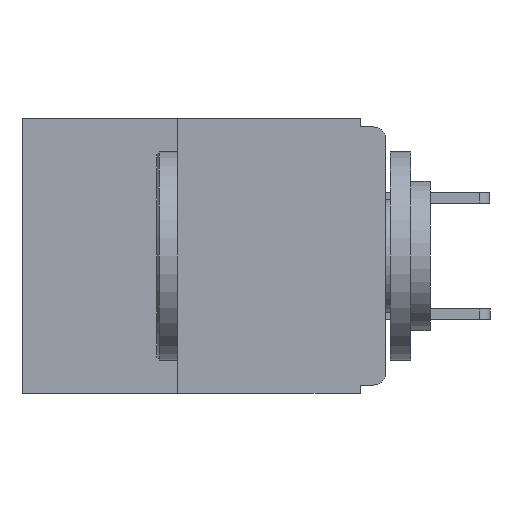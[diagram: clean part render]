
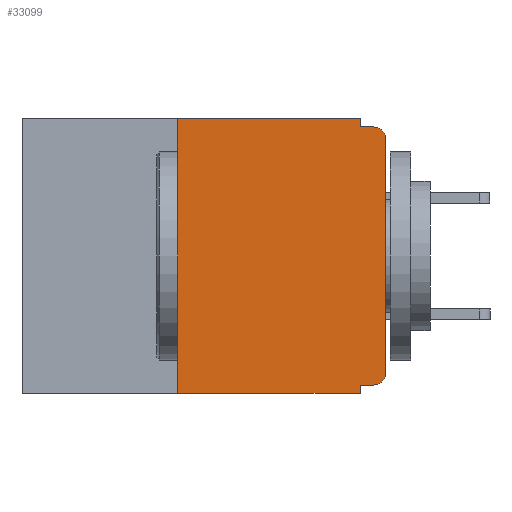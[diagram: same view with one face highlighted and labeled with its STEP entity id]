
A CAD part, left-side view. The second image highlights one B-rep face of the part: STEP entity #33099.
In plain terms, the highlighted planar face has unit normal (-1, 0, 0).
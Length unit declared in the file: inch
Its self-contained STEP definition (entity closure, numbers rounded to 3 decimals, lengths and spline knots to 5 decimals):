
#1001 = EDGE_CURVE ( 'NONE', #16274, #11754, #8063, .T. ) ;
#1783 = EDGE_CURVE ( 'NONE', #30344, #3031, #2550, .T. ) ;
#2550 = LINE ( 'NONE', #20270, #15804 ) ;
#3031 = VERTEX_POINT ( 'NONE', #18327 ) ;
#3470 = CARTESIAN_POINT ( 'NONE',  ( 0., 0.015, -0.01 ) ) ;
#3698 = AXIS2_PLACEMENT_3D ( 'NONE', #27168, #29694, #14377 ) ;
#3861 = CARTESIAN_POINT ( 'NONE',  ( 0., 0.437, 0. ) ) ;
#4147 = EDGE_CURVE ( 'NONE', #9978, #14993, #24090, .T. ) ;
#5062 = CARTESIAN_POINT ( 'NONE',  ( 0., 0.031, 0. ) ) ;
#5225 = DIRECTION ( 'NONE',  ( 0., 0., -1. ) ) ;
#5384 = AXIS2_PLACEMENT_3D ( 'NONE', #5745, #23966, #8425 ) ;
#5745 = CARTESIAN_POINT ( 'NONE',  ( 0., 0.015, -0.025 ) ) ;
#5998 = ORIENTED_EDGE ( 'NONE', *, *, #1001, .F. ) ;
#6214 = CARTESIAN_POINT ( 'NONE',  ( 0., 0., -0.025 ) ) ;
#6384 = VERTEX_POINT ( 'NONE', #3470 ) ;
#6578 = DIRECTION ( 'NONE',  ( 0., 0., 1. ) ) ;
#6771 = CARTESIAN_POINT ( 'NONE',  ( 0., 0.25, -0.33 ) ) ;
#7118 = EDGE_CURVE ( 'NONE', #16274, #3031, #19596, .T. ) ;
#7270 = VECTOR ( 'NONE', #7947, 39.37008 ) ;
#7947 = DIRECTION ( 'NONE',  ( 0., -1., 0. ) ) ;
#8063 = LINE ( 'NONE', #6771, #27885 ) ;
#8073 = CARTESIAN_POINT ( 'NONE',  ( 0., 0.437, -0.33 ) ) ;
#8425 = DIRECTION ( 'NONE',  ( 0., 0., -1. ) ) ;
#8981 = FACE_OUTER_BOUND ( 'NONE', #11424, .T. ) ;
#9074 = PLANE ( 'NONE',  #3698 ) ;
#9202 = CARTESIAN_POINT ( 'NONE',  ( 0., 0., -0.01 ) ) ;
#9669 = ORIENTED_EDGE ( 'NONE', *, *, #1783, .F. ) ;
#9970 = ORIENTED_EDGE ( 'NONE', *, *, #19701, .F. ) ;
#9978 = VERTEX_POINT ( 'NONE', #21602 ) ;
#10659 = CARTESIAN_POINT ( 'NONE',  ( 0., 0.031, -0.01 ) ) ;
#10823 = ORIENTED_EDGE ( 'NONE', *, *, #16907, .F. ) ;
#11361 = CARTESIAN_POINT ( 'NONE',  ( 0., 0.25, -0.33 ) ) ;
#11424 = EDGE_LOOP ( 'NONE', ( #22584, #19668, #19854, #10823, #9970, #5998, #25876, #9669, #19795, #16923 ) ) ;
#11754 = VERTEX_POINT ( 'NONE', #23821 ) ;
#11863 = DIRECTION ( 'NONE',  ( 0., -1., 0. ) ) ;
#12833 = DIRECTION ( 'NONE',  ( 0., 0., -1. ) ) ;
#12923 = EDGE_CURVE ( 'NONE', #19002, #6384, #29881, .T. ) ;
#13034 = DIRECTION ( 'NONE',  ( -1., 0., 0. ) ) ;
#13117 = CARTESIAN_POINT ( 'NONE',  ( 0., 0.015, -0.305 ) ) ;
#14040 = AXIS2_PLACEMENT_3D ( 'NONE', #13117, #13034, #12833 ) ;
#14279 = VECTOR ( 'NONE', #24736, 39.37008 ) ;
#14377 = DIRECTION ( 'NONE',  ( 0., 0., -1. ) ) ;
#14934 = LINE ( 'NONE', #19473, #26958 ) ;
#14993 = VERTEX_POINT ( 'NONE', #24313 ) ;
#15804 = VECTOR ( 'NONE', #5225, 39.37008 ) ;
#16274 = VERTEX_POINT ( 'NONE', #11361 ) ;
#16332 = EDGE_CURVE ( 'NONE', #9978, #30344, #14934, .T. ) ;
#16899 = LINE ( 'NONE', #21670, #22177 ) ;
#16907 = EDGE_CURVE ( 'NONE', #28744, #32203, #16899, .T. ) ;
#16923 = ORIENTED_EDGE ( 'NONE', *, *, #4147, .T. ) ;
#17728 = EDGE_CURVE ( 'NONE', #32203, #6384, #32751, .T. ) ;
#18327 = CARTESIAN_POINT ( 'NONE',  ( 0., 0.031, -0.33 ) ) ;
#19002 = VERTEX_POINT ( 'NONE', #6214 ) ;
#19473 = CARTESIAN_POINT ( 'NONE',  ( 0., 0., -0.32 ) ) ;
#19596 = LINE ( 'NONE', #8073, #7270 ) ;
#19668 = ORIENTED_EDGE ( 'NONE', *, *, #12923, .T. ) ;
#19701 = EDGE_CURVE ( 'NONE', #11754, #28744, #32994, .T. ) ;
#19795 = ORIENTED_EDGE ( 'NONE', *, *, #16332, .F. ) ;
#19854 = ORIENTED_EDGE ( 'NONE', *, *, #17728, .F. ) ;
#20270 = CARTESIAN_POINT ( 'NONE',  ( 0., 0.031, -0.33 ) ) ;
#20332 = DIRECTION ( 'NONE',  ( 0., 0., 1. ) ) ;
#21602 = CARTESIAN_POINT ( 'NONE',  ( 0., 0.015, -0.32 ) ) ;
#21670 = CARTESIAN_POINT ( 'NONE',  ( 0., 0.031, 0. ) ) ;
#22040 = DIRECTION ( 'NONE',  ( 0., 1., 0. ) ) ;
#22177 = VECTOR ( 'NONE', #24190, 39.37008 ) ;
#22584 = ORIENTED_EDGE ( 'NONE', *, *, #25483, .T. ) ;
#23821 = CARTESIAN_POINT ( 'NONE',  ( 0., 0.25, 0. ) ) ;
#23966 = DIRECTION ( 'NONE',  ( -1., 0., 0. ) ) ;
#24090 = CIRCLE ( 'NONE', #14040, 0.015 ) ;
#24190 = DIRECTION ( 'NONE',  ( 0., 0., -1. ) ) ;
#24313 = CARTESIAN_POINT ( 'NONE',  ( 0., 0., -0.305 ) ) ;
#24736 = DIRECTION ( 'NONE',  ( 0., -1., 0. ) ) ;
#25483 = EDGE_CURVE ( 'NONE', #14993, #19002, #32479, .T. ) ;
#25876 = ORIENTED_EDGE ( 'NONE', *, *, #7118, .T. ) ;
#26578 = VECTOR ( 'NONE', #20332, 39.37008 ) ;
#26958 = VECTOR ( 'NONE', #22040, 39.37008 ) ;
#27168 = CARTESIAN_POINT ( 'NONE',  ( 0., 0.437, 0. ) ) ;
#27885 = VECTOR ( 'NONE', #6578, 39.37008 ) ;
#28744 = VERTEX_POINT ( 'NONE', #5062 ) ;
#29425 = CARTESIAN_POINT ( 'NONE',  ( 0., 0.031, -0.32 ) ) ;
#29694 = DIRECTION ( 'NONE',  ( 1., 0., 0. ) ) ;
#29881 = CIRCLE ( 'NONE', #5384, 0.015 ) ;
#30344 = VERTEX_POINT ( 'NONE', #29425 ) ;
#31200 = VECTOR ( 'NONE', #11863, 39.37008 ) ;
#32203 = VERTEX_POINT ( 'NONE', #10659 ) ;
#32479 = LINE ( 'NONE', #32907, #26578 ) ;
#32751 = LINE ( 'NONE', #9202, #31200 ) ;
#32907 = CARTESIAN_POINT ( 'NONE',  ( 0., 0., 0. ) ) ;
#32994 = LINE ( 'NONE', #3861, #14279 ) ;
#33099 = ADVANCED_FACE ( 'NONE', ( #8981 ), #9074, .F. ) ;
